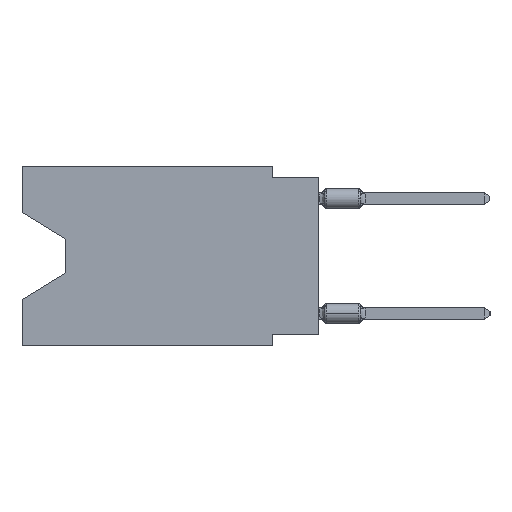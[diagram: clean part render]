
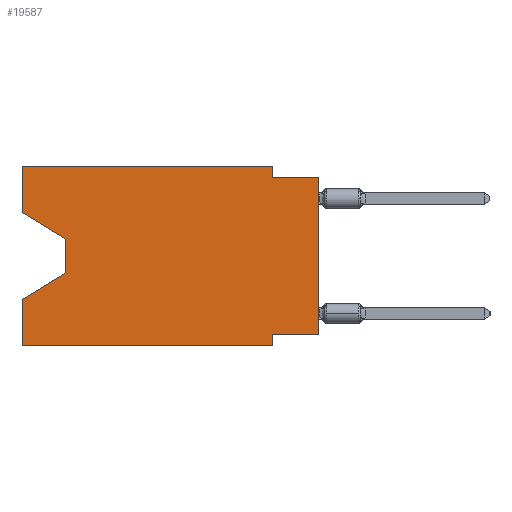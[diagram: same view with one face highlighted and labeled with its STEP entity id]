
A CAD part, left-side view. The second image highlights one B-rep face of the part: STEP entity #19587.
In plain terms, the highlighted planar face has unit normal (-1, 0, 0).
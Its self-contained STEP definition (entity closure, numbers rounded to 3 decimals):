
#36 = VECTOR ( 'NONE', #22812, 1000. ) ;
#555 = LINE ( 'NONE', #31910, #24822 ) ;
#688 = CARTESIAN_POINT ( 'NONE',  ( 0., 16.383, 0. ) ) ;
#863 = CARTESIAN_POINT ( 'NONE',  ( 0., 16.383, -9.906 ) ) ;
#2153 = CARTESIAN_POINT ( 'NONE',  ( 0., 16.383, 0. ) ) ;
#3348 = CARTESIAN_POINT ( 'NONE',  ( 0., 13.97, -4.013 ) ) ;
#3430 = VECTOR ( 'NONE', #27213, 1000. ) ;
#3580 = DIRECTION ( 'NONE',  ( 0., -1., 0. ) ) ;
#3999 = LINE ( 'NONE', #863, #5425 ) ;
#5066 = DIRECTION ( 'NONE',  ( 1., 0., 0. ) ) ;
#5068 = VECTOR ( 'NONE', #28420, 1000. ) ;
#5237 = CARTESIAN_POINT ( 'NONE',  ( 0., 2.54, 0. ) ) ;
#5425 = VECTOR ( 'NONE', #3580, 1000. ) ;
#5832 = EDGE_CURVE ( 'NONE', #17818, #23968, #3999, .T. ) ;
#5916 = VECTOR ( 'NONE', #38802, 1000. ) ;
#6279 = VERTEX_POINT ( 'NONE', #9539 ) ;
#6598 = DIRECTION ( 'NONE',  ( 0., 0., -1. ) ) ;
#6904 = EDGE_CURVE ( 'NONE', #13997, #20336, #10245, .T. ) ;
#7415 = VERTEX_POINT ( 'NONE', #25779 ) ;
#7481 = LINE ( 'NONE', #39232, #3430 ) ;
#7582 = LINE ( 'NONE', #39920, #27268 ) ;
#8393 = DIRECTION ( 'NONE',  ( 0., 0., 1. ) ) ;
#9539 = CARTESIAN_POINT ( 'NONE',  ( 0., 16.383, -7.36 ) ) ;
#9963 = LINE ( 'NONE', #35282, #5916 ) ;
#10245 = LINE ( 'NONE', #32447, #26117 ) ;
#10639 = ORIENTED_EDGE ( 'NONE', *, *, #11857, .F. ) ;
#11243 = VERTEX_POINT ( 'NONE', #23786 ) ;
#11654 = ORIENTED_EDGE ( 'NONE', *, *, #21605, .F. ) ;
#11857 = EDGE_CURVE ( 'NONE', #12619, #11243, #31122, .T. ) ;
#12119 = CARTESIAN_POINT ( 'NONE',  ( 0., 0., -9.271 ) ) ;
#12619 = VERTEX_POINT ( 'NONE', #12119 ) ;
#12950 = CARTESIAN_POINT ( 'NONE',  ( 0., 16.383, -2.546 ) ) ;
#13035 = CARTESIAN_POINT ( 'NONE',  ( 0., 16.383, 0. ) ) ;
#13121 = EDGE_CURVE ( 'NONE', #30476, #7415, #21638, .T. ) ;
#13753 = ORIENTED_EDGE ( 'NONE', *, *, #13121, .F. ) ;
#13997 = VERTEX_POINT ( 'NONE', #12950 ) ;
#14018 = DIRECTION ( 'NONE',  ( 0., 0., -1. ) ) ;
#15439 = CARTESIAN_POINT ( 'NONE',  ( 0., 16.383, 0. ) ) ;
#15645 = DIRECTION ( 'NONE',  ( 0., -1., 0. ) ) ;
#15911 = CARTESIAN_POINT ( 'NONE',  ( 0., 13.97, -5.893 ) ) ;
#16407 = EDGE_CURVE ( 'NONE', #20336, #23645, #35044, .T. ) ;
#16472 = LINE ( 'NONE', #688, #29215 ) ;
#16848 = EDGE_CURVE ( 'NONE', #36185, #30476, #16472, .T. ) ;
#17637 = ORIENTED_EDGE ( 'NONE', *, *, #27212, .T. ) ;
#17818 = VERTEX_POINT ( 'NONE', #36078 ) ;
#18372 = CARTESIAN_POINT ( 'NONE',  ( 0., 16.383, 0. ) ) ;
#19159 = ORIENTED_EDGE ( 'NONE', *, *, #6904, .T. ) ;
#19587 = ADVANCED_FACE ( 'NONE', ( #30616 ), #30005, .F. ) ;
#19905 = VECTOR ( 'NONE', #6598, 1000. ) ;
#20336 = VERTEX_POINT ( 'NONE', #3348 ) ;
#21011 = EDGE_CURVE ( 'NONE', #13997, #36185, #22082, .T. ) ;
#21390 = AXIS2_PLACEMENT_3D ( 'NONE', #2153, #5066, #14018 ) ;
#21605 = EDGE_CURVE ( 'NONE', #11243, #23968, #7481, .T. ) ;
#21638 = LINE ( 'NONE', #5237, #29002 ) ;
#21647 = ORIENTED_EDGE ( 'NONE', *, *, #33117, .F. ) ;
#21913 = CARTESIAN_POINT ( 'NONE',  ( 0., 2.54, 0. ) ) ;
#22082 = LINE ( 'NONE', #15439, #34528 ) ;
#22164 = DIRECTION ( 'NONE',  ( 0., 0.855, -0.519 ) ) ;
#22812 = DIRECTION ( 'NONE',  ( 0., 0., 1. ) ) ;
#22926 = DIRECTION ( 'NONE',  ( 0., -0.855, -0.519 ) ) ;
#23645 = VERTEX_POINT ( 'NONE', #15911 ) ;
#23723 = ORIENTED_EDGE ( 'NONE', *, *, #21011, .F. ) ;
#23786 = CARTESIAN_POINT ( 'NONE',  ( 0., 2.54, -9.271 ) ) ;
#23968 = VERTEX_POINT ( 'NONE', #28325 ) ;
#24822 = VECTOR ( 'NONE', #22164, 1000. ) ;
#25779 = CARTESIAN_POINT ( 'NONE',  ( 0., 2.54, -0.635 ) ) ;
#26117 = VECTOR ( 'NONE', #22926, 1000. ) ;
#26121 = ORIENTED_EDGE ( 'NONE', *, *, #16407, .T. ) ;
#27212 = EDGE_CURVE ( 'NONE', #23645, #6279, #555, .T. ) ;
#27213 = DIRECTION ( 'NONE',  ( 0., 0., -1. ) ) ;
#27268 = VECTOR ( 'NONE', #8393, 1000. ) ;
#28014 = CARTESIAN_POINT ( 'NONE',  ( 0., 0., -9.271 ) ) ;
#28112 = DIRECTION ( 'NONE',  ( 0., 0., 1. ) ) ;
#28325 = CARTESIAN_POINT ( 'NONE',  ( 0., 2.54, -9.906 ) ) ;
#28420 = DIRECTION ( 'NONE',  ( 0., 1., 0. ) ) ;
#29002 = VECTOR ( 'NONE', #34281, 1000. ) ;
#29215 = VECTOR ( 'NONE', #15645, 1000. ) ;
#29655 = LINE ( 'NONE', #13035, #36 ) ;
#30005 = PLANE ( 'NONE',  #21390 ) ;
#30476 = VERTEX_POINT ( 'NONE', #21913 ) ;
#30616 = FACE_OUTER_BOUND ( 'NONE', #31354, .T. ) ;
#31122 = LINE ( 'NONE', #28014, #5068 ) ;
#31354 = EDGE_LOOP ( 'NONE', ( #19159, #26121, #17637, #21647, #39887, #11654, #10639, #34571, #32039, #13753, #31747, #23723 ) ) ;
#31747 = ORIENTED_EDGE ( 'NONE', *, *, #16848, .F. ) ;
#31910 = CARTESIAN_POINT ( 'NONE',  ( 0., 13.97, -5.893 ) ) ;
#32039 = ORIENTED_EDGE ( 'NONE', *, *, #40972, .F. ) ;
#32447 = CARTESIAN_POINT ( 'NONE',  ( 0., 16.383, -2.546 ) ) ;
#33117 = EDGE_CURVE ( 'NONE', #17818, #6279, #29655, .T. ) ;
#33653 = EDGE_CURVE ( 'NONE', #12619, #34500, #7582, .T. ) ;
#34281 = DIRECTION ( 'NONE',  ( 0., 0., -1. ) ) ;
#34500 = VERTEX_POINT ( 'NONE', #40940 ) ;
#34528 = VECTOR ( 'NONE', #28112, 1000. ) ;
#34571 = ORIENTED_EDGE ( 'NONE', *, *, #33653, .T. ) ;
#35044 = LINE ( 'NONE', #37940, #19905 ) ;
#35282 = CARTESIAN_POINT ( 'NONE',  ( 0., 0., -0.635 ) ) ;
#36078 = CARTESIAN_POINT ( 'NONE',  ( 0., 16.383, -9.906 ) ) ;
#36185 = VERTEX_POINT ( 'NONE', #18372 ) ;
#37940 = CARTESIAN_POINT ( 'NONE',  ( 0., 13.97, -4.013 ) ) ;
#38802 = DIRECTION ( 'NONE',  ( 0., -1., 0. ) ) ;
#39232 = CARTESIAN_POINT ( 'NONE',  ( 0., 2.54, -9.906 ) ) ;
#39887 = ORIENTED_EDGE ( 'NONE', *, *, #5832, .T. ) ;
#39920 = CARTESIAN_POINT ( 'NONE',  ( 0., 0., 0. ) ) ;
#40940 = CARTESIAN_POINT ( 'NONE',  ( 0., 0., -0.635 ) ) ;
#40972 = EDGE_CURVE ( 'NONE', #7415, #34500, #9963, .T. ) ;
